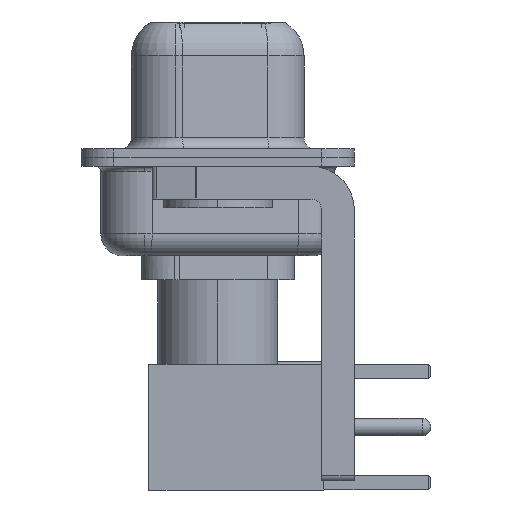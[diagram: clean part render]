
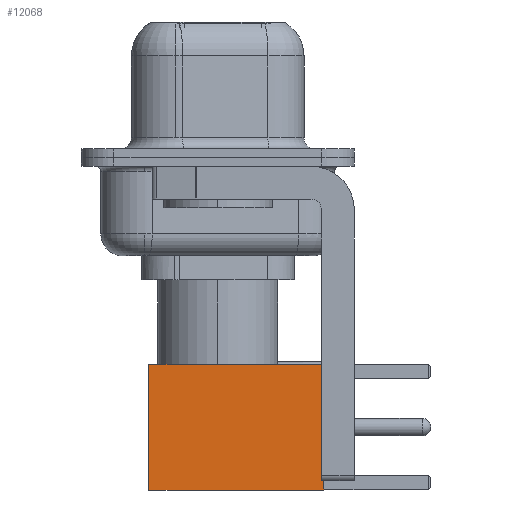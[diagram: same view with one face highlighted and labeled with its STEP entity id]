
A CAD part, left-side view. The second image highlights one B-rep face of the part: STEP entity #12068.
In plain terms, the highlighted face is planar.
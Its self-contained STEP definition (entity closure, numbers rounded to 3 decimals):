
#673 = VECTOR ( 'NONE', #21194, 1000. ) ;
#992 = LINE ( 'NONE', #4543, #12916 ) ;
#2223 = EDGE_LOOP ( 'NONE', ( #7702, #12336, #7030, #5081 ) ) ;
#2286 = LINE ( 'NONE', #23091, #673 ) ;
#2926 = CARTESIAN_POINT ( 'NONE',  ( 2.875, 2.875, 8. ) ) ;
#3486 = EDGE_CURVE ( 'NONE', #6807, #20842, #2286, .T. ) ;
#3675 = VERTEX_POINT ( 'NONE', #3975 ) ;
#3975 = CARTESIAN_POINT ( 'NONE',  ( -2.875, 2.875, 8. ) ) ;
#4343 = EDGE_CURVE ( 'NONE', #6807, #3675, #20044, .T. ) ;
#4543 = CARTESIAN_POINT ( 'NONE',  ( 0., 2.875, 0. ) ) ;
#5081 = ORIENTED_EDGE ( 'NONE', *, *, #4343, .F. ) ;
#6126 = CARTESIAN_POINT ( 'NONE',  ( 0., 2.875, 8. ) ) ;
#6792 = LINE ( 'NONE', #14581, #14395 ) ;
#6807 = VERTEX_POINT ( 'NONE', #2926 ) ;
#7030 = ORIENTED_EDGE ( 'NONE', *, *, #16475, .F. ) ;
#7702 = ORIENTED_EDGE ( 'NONE', *, *, #3486, .T. ) ;
#9518 = CARTESIAN_POINT ( 'NONE',  ( -2.875, 2.875, 0. ) ) ;
#12068 = ADVANCED_FACE ( 'NONE', ( #15279 ), #19134, .T. ) ;
#12116 = DIRECTION ( 'NONE',  ( -1., 0., 0. ) ) ;
#12336 = ORIENTED_EDGE ( 'NONE', *, *, #12660, .T. ) ;
#12660 = EDGE_CURVE ( 'NONE', #20842, #25040, #992, .T. ) ;
#12916 = VECTOR ( 'NONE', #14774, 1000. ) ;
#14395 = VECTOR ( 'NONE', #20580, 1000. ) ;
#14581 = CARTESIAN_POINT ( 'NONE',  ( -2.875, 2.875, 0. ) ) ;
#14774 = DIRECTION ( 'NONE',  ( -1., 0., 0. ) ) ;
#15279 = FACE_OUTER_BOUND ( 'NONE', #2223, .T. ) ;
#15392 = VECTOR ( 'NONE', #12116, 1000. ) ;
#16475 = EDGE_CURVE ( 'NONE', #3675, #25040, #6792, .T. ) ;
#18252 = CARTESIAN_POINT ( 'NONE',  ( 2.875, 2.875, 0. ) ) ;
#18913 = AXIS2_PLACEMENT_3D ( 'NONE', #19385, #22928, #21037 ) ;
#19134 = PLANE ( 'NONE',  #18913 ) ;
#19385 = CARTESIAN_POINT ( 'NONE',  ( 2.875, 2.875, 0. ) ) ;
#20044 = LINE ( 'NONE', #6126, #15392 ) ;
#20580 = DIRECTION ( 'NONE',  ( 0., 0., -1. ) ) ;
#20842 = VERTEX_POINT ( 'NONE', #18252 ) ;
#21037 = DIRECTION ( 'NONE',  ( 0., 0., 1. ) ) ;
#21194 = DIRECTION ( 'NONE',  ( 0., 0., -1. ) ) ;
#22928 = DIRECTION ( 'NONE',  ( 0., 1., 0. ) ) ;
#23091 = CARTESIAN_POINT ( 'NONE',  ( 2.875, 2.875, 0. ) ) ;
#25040 = VERTEX_POINT ( 'NONE', #9518 ) ;
